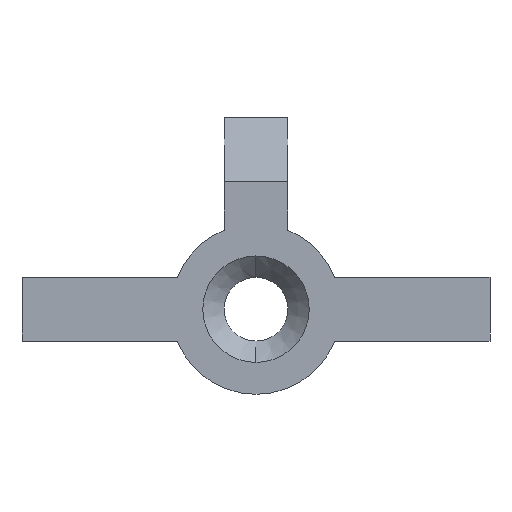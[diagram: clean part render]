
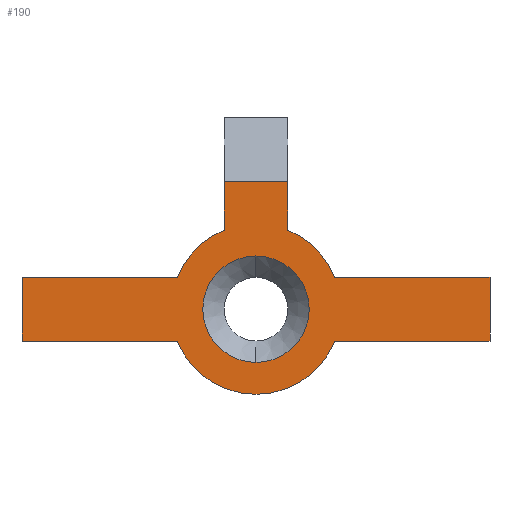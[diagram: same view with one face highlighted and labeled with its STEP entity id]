
A CAD part, front view. The second image highlights one B-rep face of the part: STEP entity #190.
In plain terms, the highlighted planar face has unit normal (0, -1, 0).
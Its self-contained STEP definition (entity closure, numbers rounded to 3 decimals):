
#8 = VECTOR ( 'NONE', #627, 1000. ) ;
#10 = DIRECTION ( 'NONE',  ( 0., 0., -1. ) ) ;
#11 = CARTESIAN_POINT ( 'NONE',  ( 11., -25., -9. ) ) ;
#19 = DIRECTION ( 'NONE',  ( 0., 1., 0. ) ) ;
#21 = VECTOR ( 'NONE', #636, 1000. ) ;
#23 = CARTESIAN_POINT ( 'NONE',  ( 0., -25., -7.5 ) ) ;
#27 = LINE ( 'NONE', #633, #8 ) ;
#32 = VECTOR ( 'NONE', #80, 1000. ) ;
#33 = DIRECTION ( 'NONE',  ( 1., 0., 0. ) ) ;
#37 = VERTEX_POINT ( 'NONE', #602 ) ;
#39 = CARTESIAN_POINT ( 'NONE',  ( 11., -25., -9. ) ) ;
#40 = FACE_BOUND ( 'NONE', #643, .T. ) ;
#43 = DIRECTION ( 'NONE',  ( 0., 0., -1. ) ) ;
#44 = VERTEX_POINT ( 'NONE', #100 ) ;
#51 = VERTEX_POINT ( 'NONE', #59 ) ;
#52 = VECTOR ( 'NONE', #33, 1000. ) ;
#54 = FACE_OUTER_BOUND ( 'NONE', #622, .T. ) ;
#58 = DIRECTION ( 'NONE',  ( 0., 0., -1. ) ) ;
#59 = CARTESIAN_POINT ( 'NONE',  ( 3.708, -25., -9. ) ) ;
#60 = DIRECTION ( 'NONE',  ( 0., 1., 0. ) ) ;
#63 = CARTESIAN_POINT ( 'NONE',  ( 0., -25., -7.5 ) ) ;
#65 = LINE ( 'NONE', #641, #21 ) ;
#77 = VERTEX_POINT ( 'NONE', #388 ) ;
#79 = LINE ( 'NONE', #39, #52 ) ;
#80 = DIRECTION ( 'NONE',  ( 1., 0., 0. ) ) ;
#82 = CARTESIAN_POINT ( 'NONE',  ( 11., -25., -9. ) ) ;
#83 = VERTEX_POINT ( 'NONE', #443 ) ;
#84 = VECTOR ( 'NONE', #90, 1000. ) ;
#90 = DIRECTION ( 'NONE',  ( -1., 0., 0. ) ) ;
#91 = VERTEX_POINT ( 'NONE', #447 ) ;
#98 = LINE ( 'NONE', #245, #84 ) ;
#100 = CARTESIAN_POINT ( 'NONE',  ( -1.5, -25., -3.792 ) ) ;
#102 = DIRECTION ( 'NONE',  ( 0., 0., -1. ) ) ;
#108 = LINE ( 'NONE', #82, #32 ) ;
#110 = VERTEX_POINT ( 'NONE', #275 ) ;
#111 = DIRECTION ( 'NONE',  ( 0., -1., 0. ) ) ;
#113 = VECTOR ( 'NONE', #120, 1000. ) ;
#119 = LINE ( 'NONE', #306, #165 ) ;
#120 = DIRECTION ( 'NONE',  ( 0., 0., -1. ) ) ;
#123 = VECTOR ( 'NONE', #234, 1000. ) ;
#128 = CARTESIAN_POINT ( 'NONE',  ( 0., -25., -7.5 ) ) ;
#130 = VERTEX_POINT ( 'NONE', #203 ) ;
#132 = LINE ( 'NONE', #171, #113 ) ;
#139 = VECTOR ( 'NONE', #530, 1000. ) ;
#146 = LINE ( 'NONE', #295, #123 ) ;
#165 = VECTOR ( 'NONE', #43, 1000. ) ;
#171 = CARTESIAN_POINT ( 'NONE',  ( -1.5, -25., 1.5 ) ) ;
#186 = VERTEX_POINT ( 'NONE', #542 ) ;
#190 = ADVANCED_FACE ( 'NONE', ( #40, #54 ), #429, .T. ) ;
#191 = VERTEX_POINT ( 'NONE', #488 ) ;
#200 = LINE ( 'NONE', #361, #139 ) ;
#203 = CARTESIAN_POINT ( 'NONE',  ( 0., -25., -11.5 ) ) ;
#230 = AXIS2_PLACEMENT_3D ( 'NONE', #252, #248, #239 ) ;
#234 = DIRECTION ( 'NONE',  ( -1., 0., 0. ) ) ;
#239 = DIRECTION ( 'NONE',  ( 0., 0., -1. ) ) ;
#245 = CARTESIAN_POINT ( 'NONE',  ( 11., -25., -6. ) ) ;
#248 = DIRECTION ( 'NONE',  ( 0., -1., 0. ) ) ;
#252 = CARTESIAN_POINT ( 'NONE',  ( 0., -25., -7.5 ) ) ;
#257 = AXIS2_PLACEMENT_3D ( 'NONE', #23, #19, #10 ) ;
#265 = AXIS2_PLACEMENT_3D ( 'NONE', #63, #60, #58 ) ;
#267 = AXIS2_PLACEMENT_3D ( 'NONE', #128, #111, #102 ) ;
#275 = CARTESIAN_POINT ( 'NONE',  ( 1.5, -25., -3.792 ) ) ;
#279 = AXIS2_PLACEMENT_3D ( 'NONE', #389, #383, #377 ) ;
#281 = AXIS2_PLACEMENT_3D ( 'NONE', #401, #397, #395 ) ;
#284 = VERTEX_POINT ( 'NONE', #11 ) ;
#291 = CARTESIAN_POINT ( 'NONE',  ( 11., -25., -6. ) ) ;
#295 = CARTESIAN_POINT ( 'NONE',  ( 0., -25., -1.5 ) ) ;
#306 = CARTESIAN_POINT ( 'NONE',  ( -11., -25., -6. ) ) ;
#327 = CIRCLE ( 'NONE', #257, 2.5 ) ;
#351 = VERTEX_POINT ( 'NONE', #567 ) ;
#361 = CARTESIAN_POINT ( 'NONE',  ( 1.5, -25., 1.5 ) ) ;
#362 = AXIS2_PLACEMENT_3D ( 'NONE', #505, #442, #450 ) ;
#363 = ORIENTED_EDGE ( 'NONE', *, *, #423, .T. ) ;
#373 = ORIENTED_EDGE ( 'NONE', *, *, #435, .T. ) ;
#377 = DIRECTION ( 'NONE',  ( 0., 0., -1. ) ) ;
#378 = CIRCLE ( 'NONE', #265, 2.5 ) ;
#383 = DIRECTION ( 'NONE',  ( 0., -1., 0. ) ) ;
#388 = CARTESIAN_POINT ( 'NONE',  ( -1.5, -25., -1.5 ) ) ;
#389 = CARTESIAN_POINT ( 'NONE',  ( 0., -25., -7.5 ) ) ;
#390 = VERTEX_POINT ( 'NONE', #509 ) ;
#393 = EDGE_CURVE ( 'NONE', #44, #83, #517, .T. ) ;
#395 = DIRECTION ( 'NONE',  ( 0., 0., -1. ) ) ;
#396 = EDGE_CURVE ( 'NONE', #130, #51, #647, .T. ) ;
#397 = DIRECTION ( 'NONE',  ( 0., -1., 0. ) ) ;
#401 = CARTESIAN_POINT ( 'NONE',  ( 0., -25., -7.5 ) ) ;
#406 = ORIENTED_EDGE ( 'NONE', *, *, #464, .T. ) ;
#413 = ORIENTED_EDGE ( 'NONE', *, *, #466, .T. ) ;
#417 = EDGE_CURVE ( 'NONE', #37, #130, #452, .T. ) ;
#423 = EDGE_CURVE ( 'NONE', #186, #191, #378, .T. ) ;
#425 = ORIENTED_EDGE ( 'NONE', *, *, #467, .T. ) ;
#427 = ORIENTED_EDGE ( 'NONE', *, *, #393, .T. ) ;
#429 = PLANE ( 'NONE',  #362 ) ;
#435 = EDGE_CURVE ( 'NONE', #191, #186, #327, .T. ) ;
#436 = ORIENTED_EDGE ( 'NONE', *, *, #473, .T. ) ;
#442 = DIRECTION ( 'NONE',  ( 0., -1., 0. ) ) ;
#443 = CARTESIAN_POINT ( 'NONE',  ( -3.708, -25., -6. ) ) ;
#447 = CARTESIAN_POINT ( 'NONE',  ( 3.708, -25., -6. ) ) ;
#450 = DIRECTION ( 'NONE',  ( 0., 0., -1. ) ) ;
#452 = CIRCLE ( 'NONE', #267, 4. ) ;
#455 = ORIENTED_EDGE ( 'NONE', *, *, #475, .T. ) ;
#464 = EDGE_CURVE ( 'NONE', #110, #390, #200, .T. ) ;
#466 = EDGE_CURVE ( 'NONE', #390, #77, #146, .T. ) ;
#467 = EDGE_CURVE ( 'NONE', #77, #44, #132, .T. ) ;
#473 = EDGE_CURVE ( 'NONE', #83, #519, #98, .T. ) ;
#475 = EDGE_CURVE ( 'NONE', #519, #351, #119, .T. ) ;
#478 = EDGE_CURVE ( 'NONE', #351, #37, #79, .T. ) ;
#480 = CIRCLE ( 'NONE', #230, 4. ) ;
#482 = ORIENTED_EDGE ( 'NONE', *, *, #478, .T. ) ;
#483 = EDGE_CURVE ( 'NONE', #51, #284, #108, .T. ) ;
#484 = EDGE_CURVE ( 'NONE', #284, #632, #65, .T. ) ;
#487 = EDGE_CURVE ( 'NONE', #632, #91, #27, .T. ) ;
#488 = CARTESIAN_POINT ( 'NONE',  ( 0., -25., -5. ) ) ;
#493 = ORIENTED_EDGE ( 'NONE', *, *, #417, .T. ) ;
#505 = CARTESIAN_POINT ( 'NONE',  ( 0., -25., -7.5 ) ) ;
#509 = CARTESIAN_POINT ( 'NONE',  ( 1.5, -25., -1.5 ) ) ;
#511 = ORIENTED_EDGE ( 'NONE', *, *, #396, .T. ) ;
#512 = ORIENTED_EDGE ( 'NONE', *, *, #483, .T. ) ;
#517 = CIRCLE ( 'NONE', #281, 4. ) ;
#519 = VERTEX_POINT ( 'NONE', #526 ) ;
#526 = CARTESIAN_POINT ( 'NONE',  ( -11., -25., -6. ) ) ;
#527 = ORIENTED_EDGE ( 'NONE', *, *, #484, .T. ) ;
#530 = DIRECTION ( 'NONE',  ( 0., 0., 1. ) ) ;
#533 = ORIENTED_EDGE ( 'NONE', *, *, #487, .T. ) ;
#542 = CARTESIAN_POINT ( 'NONE',  ( 0., -25., -10. ) ) ;
#544 = ORIENTED_EDGE ( 'NONE', *, *, #551, .T. ) ;
#551 = EDGE_CURVE ( 'NONE', #91, #110, #480, .T. ) ;
#567 = CARTESIAN_POINT ( 'NONE',  ( -11., -25., -9. ) ) ;
#602 = CARTESIAN_POINT ( 'NONE',  ( -3.708, -25., -9. ) ) ;
#622 = EDGE_LOOP ( 'NONE', ( #406, #413, #425, #427, #436, #455, #482, #493, #511, #512, #527, #533, #544 ) ) ;
#627 = DIRECTION ( 'NONE',  ( -1., 0., 0. ) ) ;
#632 = VERTEX_POINT ( 'NONE', #291 ) ;
#633 = CARTESIAN_POINT ( 'NONE',  ( 11., -25., -6. ) ) ;
#636 = DIRECTION ( 'NONE',  ( 0., 0., 1. ) ) ;
#641 = CARTESIAN_POINT ( 'NONE',  ( 11., -25., -6. ) ) ;
#643 = EDGE_LOOP ( 'NONE', ( #363, #373 ) ) ;
#647 = CIRCLE ( 'NONE', #279, 4. ) ;
